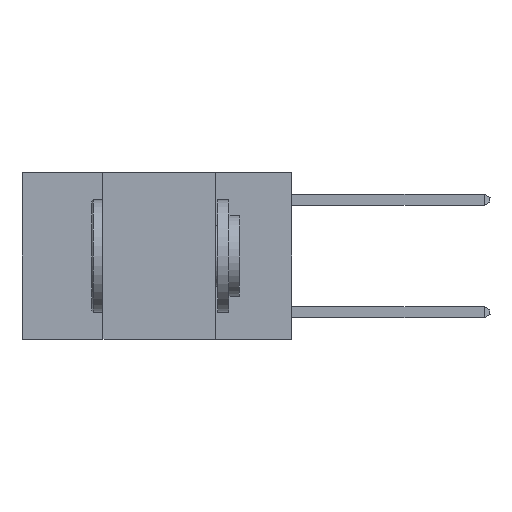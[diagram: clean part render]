
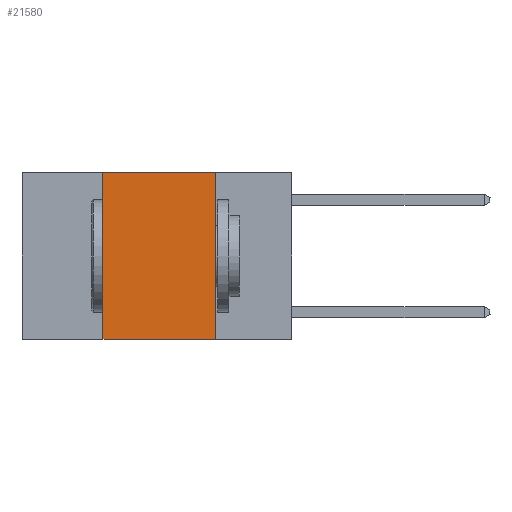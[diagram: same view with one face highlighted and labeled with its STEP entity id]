
A CAD part, left-side view. The second image highlights one B-rep face of the part: STEP entity #21580.
In plain terms, the highlighted planar face has unit normal (-1, 0, 0).
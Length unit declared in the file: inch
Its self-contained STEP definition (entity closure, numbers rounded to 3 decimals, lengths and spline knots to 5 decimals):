
#1747 = CARTESIAN_POINT ( 'NONE',  ( 0., 0.42, 0. ) ) ;
#1813 = VECTOR ( 'NONE', #6593, 39.37008 ) ;
#1925 = DIRECTION ( 'NONE',  ( 0., -1., 0. ) ) ;
#2860 = VECTOR ( 'NONE', #19181, 39.37008 ) ;
#3460 = EDGE_CURVE ( 'NONE', #10508, #12414, #16361, .T. ) ;
#4264 = VECTOR ( 'NONE', #23581, 39.37008 ) ;
#4843 = DIRECTION ( 'NONE',  ( 1., 0., 0. ) ) ;
#5084 = LINE ( 'NONE', #12801, #23164 ) ;
#5095 = ORIENTED_EDGE ( 'NONE', *, *, #10147, .F. ) ;
#6593 = DIRECTION ( 'NONE',  ( 0., 0., -1. ) ) ;
#8011 = CARTESIAN_POINT ( 'NONE',  ( 0., 0.42, -0.37 ) ) ;
#8498 = CARTESIAN_POINT ( 'NONE',  ( 0., 0.6, 0. ) ) ;
#10147 = EDGE_CURVE ( 'NONE', #13375, #10508, #5084, .T. ) ;
#10508 = VERTEX_POINT ( 'NONE', #14434 ) ;
#10829 = ORIENTED_EDGE ( 'NONE', *, *, #22115, .F. ) ;
#12397 = EDGE_LOOP ( 'NONE', ( #15009, #5095, #10829, #22853 ) ) ;
#12414 = VERTEX_POINT ( 'NONE', #20874 ) ;
#12801 = CARTESIAN_POINT ( 'NONE',  ( 0., 0.6, 0. ) ) ;
#13342 = LINE ( 'NONE', #21103, #2860 ) ;
#13375 = VERTEX_POINT ( 'NONE', #1747 ) ;
#14434 = CARTESIAN_POINT ( 'NONE',  ( 0., 0.17, 0. ) ) ;
#15009 = ORIENTED_EDGE ( 'NONE', *, *, #3460, .F. ) ;
#16361 = LINE ( 'NONE', #23987, #1813 ) ;
#16722 = LINE ( 'NONE', #19492, #4264 ) ;
#18151 = FACE_OUTER_BOUND ( 'NONE', #12397, .T. ) ;
#19181 = DIRECTION ( 'NONE',  ( 0., -1., 0. ) ) ;
#19492 = CARTESIAN_POINT ( 'NONE',  ( 0., 0.42, 0. ) ) ;
#20300 = DIRECTION ( 'NONE',  ( 0., 0., -1. ) ) ;
#20874 = CARTESIAN_POINT ( 'NONE',  ( 0., 0.17, -0.37 ) ) ;
#21103 = CARTESIAN_POINT ( 'NONE',  ( 0., 0.6, -0.37 ) ) ;
#21580 = ADVANCED_FACE ( 'NONE', ( #18151 ), #22094, .F. ) ;
#22094 = PLANE ( 'NONE',  #23829 ) ;
#22115 = EDGE_CURVE ( 'NONE', #24172, #13375, #16722, .T. ) ;
#22853 = ORIENTED_EDGE ( 'NONE', *, *, #24048, .T. ) ;
#23164 = VECTOR ( 'NONE', #1925, 39.37008 ) ;
#23581 = DIRECTION ( 'NONE',  ( 0., 0., 1. ) ) ;
#23829 = AXIS2_PLACEMENT_3D ( 'NONE', #8498, #4843, #20300 ) ;
#23987 = CARTESIAN_POINT ( 'NONE',  ( 0., 0.17, 0. ) ) ;
#24048 = EDGE_CURVE ( 'NONE', #24172, #12414, #13342, .T. ) ;
#24172 = VERTEX_POINT ( 'NONE', #8011 ) ;
